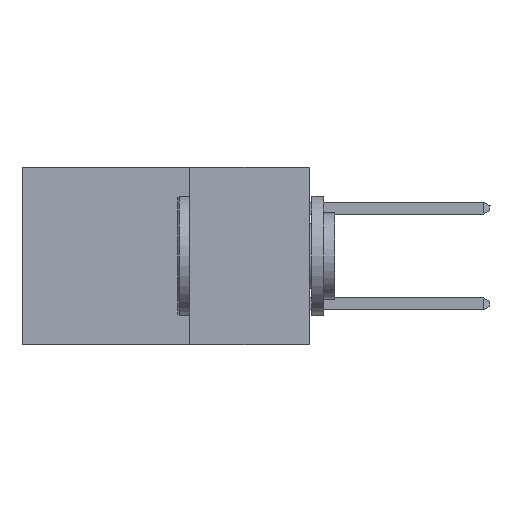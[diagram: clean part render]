
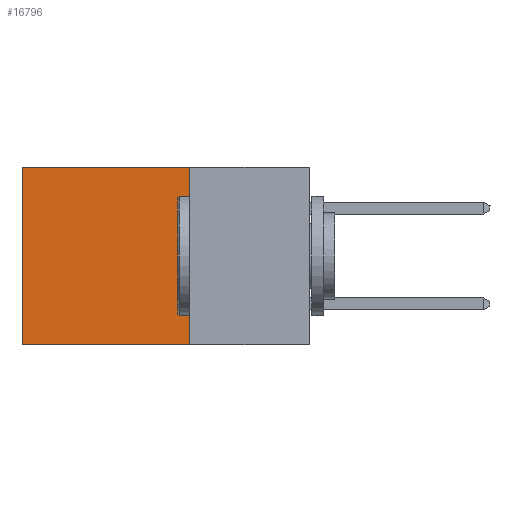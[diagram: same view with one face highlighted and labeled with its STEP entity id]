
A CAD part, left-side view. The second image highlights one B-rep face of the part: STEP entity #16796.
In plain terms, the highlighted planar face has unit normal (-1, 0, 0).
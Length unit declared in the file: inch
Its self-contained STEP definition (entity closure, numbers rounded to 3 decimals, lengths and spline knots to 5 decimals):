
#227 = AXIS2_PLACEMENT_3D ( 'NONE', #3983, #14801, #5609 ) ;
#2186 = CARTESIAN_POINT ( 'NONE',  ( 0.2875, 0.6, -0.37 ) ) ;
#2337 = ORIENTED_EDGE ( 'NONE', *, *, #13385, .T. ) ;
#2691 = DIRECTION ( 'NONE',  ( 0., 1., 0. ) ) ;
#2741 = EDGE_LOOP ( 'NONE', ( #13686, #3766, #18431, #2337 ) ) ;
#3766 = ORIENTED_EDGE ( 'NONE', *, *, #12813, .F. ) ;
#3875 = LINE ( 'NONE', #17068, #19111 ) ;
#3983 = CARTESIAN_POINT ( 'NONE',  ( 0.2875, 0.25, 0. ) ) ;
#4531 = DIRECTION ( 'NONE',  ( 0., 1., 0. ) ) ;
#4688 = FACE_OUTER_BOUND ( 'NONE', #2741, .T. ) ;
#4930 = VERTEX_POINT ( 'NONE', #15126 ) ;
#5397 = EDGE_CURVE ( 'NONE', #4930, #9062, #15883, .T. ) ;
#5609 = DIRECTION ( 'NONE',  ( 0., 0., -1. ) ) ;
#5975 = CARTESIAN_POINT ( 'NONE',  ( 0.2875, 0.25, -0.37 ) ) ;
#6227 = VERTEX_POINT ( 'NONE', #9257 ) ;
#6578 = VECTOR ( 'NONE', #2691, 39.37008 ) ;
#7248 = CARTESIAN_POINT ( 'NONE',  ( 0.2875, 0.25, 0. ) ) ;
#8761 = VECTOR ( 'NONE', #4531, 39.37008 ) ;
#9058 = CARTESIAN_POINT ( 'NONE',  ( 0.2875, 0.25, 0. ) ) ;
#9062 = VERTEX_POINT ( 'NONE', #5975 ) ;
#9257 = CARTESIAN_POINT ( 'NONE',  ( 0.2875, 0.6, 0. ) ) ;
#10715 = LINE ( 'NONE', #9058, #6578 ) ;
#11891 = VECTOR ( 'NONE', #19260, 39.37008 ) ;
#12813 = EDGE_CURVE ( 'NONE', #9062, #18942, #15604, .T. ) ;
#13311 = PLANE ( 'NONE',  #227 ) ;
#13385 = EDGE_CURVE ( 'NONE', #4930, #6227, #10715, .T. ) ;
#13686 = ORIENTED_EDGE ( 'NONE', *, *, #19802, .T. ) ;
#14801 = DIRECTION ( 'NONE',  ( 1., 0., 0. ) ) ;
#15126 = CARTESIAN_POINT ( 'NONE',  ( 0.2875, 0.25, 0. ) ) ;
#15296 = CARTESIAN_POINT ( 'NONE',  ( 0.2875, 0.25, -0.37 ) ) ;
#15604 = LINE ( 'NONE', #15296, #8761 ) ;
#15883 = LINE ( 'NONE', #7248, #11891 ) ;
#16796 = ADVANCED_FACE ( 'NONE', ( #4688 ), #13311, .F. ) ;
#17068 = CARTESIAN_POINT ( 'NONE',  ( 0.2875, 0.6, 0. ) ) ;
#18431 = ORIENTED_EDGE ( 'NONE', *, *, #5397, .F. ) ;
#18514 = DIRECTION ( 'NONE',  ( 0., 0., -1. ) ) ;
#18942 = VERTEX_POINT ( 'NONE', #2186 ) ;
#19111 = VECTOR ( 'NONE', #18514, 39.37008 ) ;
#19260 = DIRECTION ( 'NONE',  ( 0., 0., -1. ) ) ;
#19802 = EDGE_CURVE ( 'NONE', #6227, #18942, #3875, .T. ) ;
